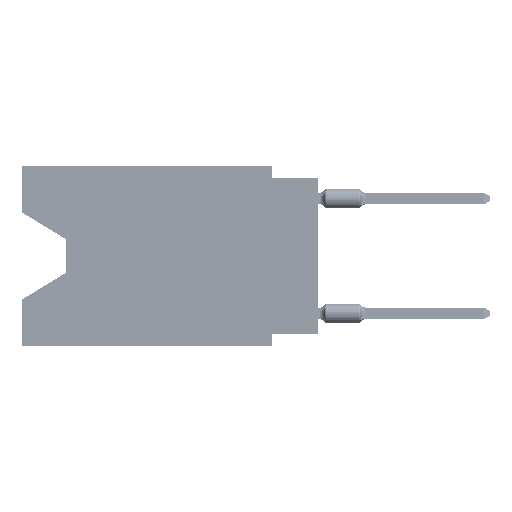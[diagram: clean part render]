
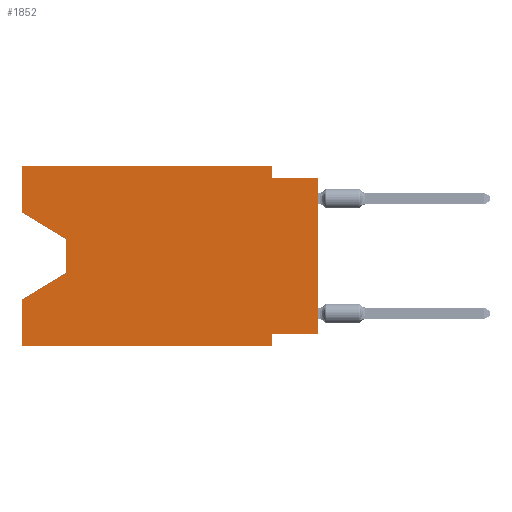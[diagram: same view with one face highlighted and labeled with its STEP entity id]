
A CAD part, left-side view. The second image highlights one B-rep face of the part: STEP entity #1852.
In plain terms, the highlighted planar face has unit normal (-1, 0, 0).
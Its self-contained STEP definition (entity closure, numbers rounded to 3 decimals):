
#822 = ORIENTED_EDGE ( 'NONE', *, *, #31095, .T. ) ;
#990 = CARTESIAN_POINT ( 'NONE',  ( 0., 16.383, 0. ) ) ;
#1060 = EDGE_CURVE ( 'NONE', #25016, #70449, #39018, .T. ) ;
#1229 = ORIENTED_EDGE ( 'NONE', *, *, #8433, .F. ) ;
#1852 = ADVANCED_FACE ( 'NONE', ( #47980 ), #70160, .F. ) ;
#2499 = ORIENTED_EDGE ( 'NONE', *, *, #43273, .F. ) ;
#2835 = EDGE_CURVE ( 'NONE', #46178, #70449, #46001, .T. ) ;
#5629 = ORIENTED_EDGE ( 'NONE', *, *, #1060, .F. ) ;
#6577 = DIRECTION ( 'NONE',  ( 0., -1., 0. ) ) ;
#7073 = EDGE_CURVE ( 'NONE', #48018, #15986, #58501, .T. ) ;
#8433 = EDGE_CURVE ( 'NONE', #41950, #25016, #15344, .T. ) ;
#8598 = VECTOR ( 'NONE', #38591, 1000. ) ;
#8704 = DIRECTION ( 'NONE',  ( 0., -1., 0. ) ) ;
#10518 = CARTESIAN_POINT ( 'NONE',  ( 0., 16.383, 0. ) ) ;
#12335 = VERTEX_POINT ( 'NONE', #43692 ) ;
#13188 = CARTESIAN_POINT ( 'NONE',  ( 0., 16.383, -2.546 ) ) ;
#13971 = ORIENTED_EDGE ( 'NONE', *, *, #64908, .F. ) ;
#14072 = CARTESIAN_POINT ( 'NONE',  ( 0., 2.54, -9.906 ) ) ;
#14372 = VERTEX_POINT ( 'NONE', #65568 ) ;
#14625 = DIRECTION ( 'NONE',  ( 0., 1., 0. ) ) ;
#14948 = CARTESIAN_POINT ( 'NONE',  ( 0., 13.97, -4.013 ) ) ;
#15196 = CARTESIAN_POINT ( 'NONE',  ( 0., 0., -9.271 ) ) ;
#15344 = LINE ( 'NONE', #53143, #36620 ) ;
#15986 = VERTEX_POINT ( 'NONE', #57147 ) ;
#16194 = ORIENTED_EDGE ( 'NONE', *, *, #7073, .F. ) ;
#17144 = ORIENTED_EDGE ( 'NONE', *, *, #54822, .T. ) ;
#17382 = DIRECTION ( 'NONE',  ( 0., 0., 1. ) ) ;
#17681 = DIRECTION ( 'NONE',  ( 0., 0., 1. ) ) ;
#18963 = VECTOR ( 'NONE', #17681, 1000. ) ;
#19224 = VECTOR ( 'NONE', #69356, 1000. ) ;
#20285 = VECTOR ( 'NONE', #48889, 1000. ) ;
#21452 = EDGE_CURVE ( 'NONE', #12335, #45288, #43662, .T. ) ;
#22569 = CARTESIAN_POINT ( 'NONE',  ( 0., 16.383, 0. ) ) ;
#22991 = CARTESIAN_POINT ( 'NONE',  ( 0., 2.54, 0. ) ) ;
#25016 = VERTEX_POINT ( 'NONE', #71754 ) ;
#25036 = VECTOR ( 'NONE', #8704, 1000. ) ;
#26215 = LINE ( 'NONE', #14948, #28585 ) ;
#27399 = ORIENTED_EDGE ( 'NONE', *, *, #30727, .T. ) ;
#28585 = VECTOR ( 'NONE', #48374, 1000. ) ;
#28944 = CARTESIAN_POINT ( 'NONE',  ( 0., 16.383, -9.906 ) ) ;
#29575 = CARTESIAN_POINT ( 'NONE',  ( 0., 2.54, -9.906 ) ) ;
#29761 = LINE ( 'NONE', #31193, #19224 ) ;
#30727 = EDGE_CURVE ( 'NONE', #41950, #15986, #54342, .T. ) ;
#31095 = EDGE_CURVE ( 'NONE', #48826, #69451, #36443, .T. ) ;
#31193 = CARTESIAN_POINT ( 'NONE',  ( 0., 13.97, -5.893 ) ) ;
#31634 = DIRECTION ( 'NONE',  ( 0., 0., -1. ) ) ;
#32834 = EDGE_CURVE ( 'NONE', #69451, #38051, #26215, .T. ) ;
#36196 = EDGE_LOOP ( 'NONE', ( #822, #46375, #17144, #2499, #64024, #5629, #1229, #27399, #16194, #13971, #56363, #38652 ) ) ;
#36443 = LINE ( 'NONE', #58630, #63208 ) ;
#36620 = VECTOR ( 'NONE', #14625, 1000. ) ;
#38051 = VERTEX_POINT ( 'NONE', #55431 ) ;
#38591 = DIRECTION ( 'NONE',  ( 0., 0., -1. ) ) ;
#38652 = ORIENTED_EDGE ( 'NONE', *, *, #53587, .F. ) ;
#39018 = LINE ( 'NONE', #29575, #42906 ) ;
#39137 = LINE ( 'NONE', #990, #18963 ) ;
#41950 = VERTEX_POINT ( 'NONE', #15196 ) ;
#42129 = CARTESIAN_POINT ( 'NONE',  ( 0., 0., -0.635 ) ) ;
#42344 = CARTESIAN_POINT ( 'NONE',  ( 0., 0., 0. ) ) ;
#42519 = CARTESIAN_POINT ( 'NONE',  ( 0., 16.383, 0. ) ) ;
#42906 = VECTOR ( 'NONE', #44831, 1000. ) ;
#43273 = EDGE_CURVE ( 'NONE', #46178, #14372, #39137, .T. ) ;
#43662 = LINE ( 'NONE', #22569, #67123 ) ;
#43692 = CARTESIAN_POINT ( 'NONE',  ( 0., 16.383, 0. ) ) ;
#43700 = LINE ( 'NONE', #60435, #8598 ) ;
#44639 = LINE ( 'NONE', #10518, #59856 ) ;
#44831 = DIRECTION ( 'NONE',  ( 0., 0., -1. ) ) ;
#45288 = VERTEX_POINT ( 'NONE', #22991 ) ;
#46001 = LINE ( 'NONE', #28944, #59492 ) ;
#46178 = VERTEX_POINT ( 'NONE', #57545 ) ;
#46375 = ORIENTED_EDGE ( 'NONE', *, *, #32834, .T. ) ;
#47980 = FACE_OUTER_BOUND ( 'NONE', #36196, .T. ) ;
#48018 = VERTEX_POINT ( 'NONE', #49649 ) ;
#48374 = DIRECTION ( 'NONE',  ( 0., 0., -1. ) ) ;
#48826 = VERTEX_POINT ( 'NONE', #13188 ) ;
#48889 = DIRECTION ( 'NONE',  ( 0., 0., 1. ) ) ;
#49649 = CARTESIAN_POINT ( 'NONE',  ( 0., 2.54, -0.635 ) ) ;
#53143 = CARTESIAN_POINT ( 'NONE',  ( 0., 0., -9.271 ) ) ;
#53587 = EDGE_CURVE ( 'NONE', #48826, #12335, #44639, .T. ) ;
#54342 = LINE ( 'NONE', #42344, #20285 ) ;
#54822 = EDGE_CURVE ( 'NONE', #38051, #14372, #29761, .T. ) ;
#55431 = CARTESIAN_POINT ( 'NONE',  ( 0., 13.97, -5.893 ) ) ;
#55803 = CARTESIAN_POINT ( 'NONE',  ( 0., 13.97, -4.013 ) ) ;
#56363 = ORIENTED_EDGE ( 'NONE', *, *, #21452, .F. ) ;
#57147 = CARTESIAN_POINT ( 'NONE',  ( 0., 0., -0.635 ) ) ;
#57545 = CARTESIAN_POINT ( 'NONE',  ( 0., 16.383, -9.906 ) ) ;
#58501 = LINE ( 'NONE', #42129, #25036 ) ;
#58630 = CARTESIAN_POINT ( 'NONE',  ( 0., 16.383, -2.546 ) ) ;
#59260 = DIRECTION ( 'NONE',  ( 1., 0., 0. ) ) ;
#59492 = VECTOR ( 'NONE', #68183, 1000. ) ;
#59856 = VECTOR ( 'NONE', #17382, 1000. ) ;
#60435 = CARTESIAN_POINT ( 'NONE',  ( 0., 2.54, 0. ) ) ;
#63208 = VECTOR ( 'NONE', #64813, 1000. ) ;
#64024 = ORIENTED_EDGE ( 'NONE', *, *, #2835, .T. ) ;
#64813 = DIRECTION ( 'NONE',  ( 0., -0.855, -0.519 ) ) ;
#64908 = EDGE_CURVE ( 'NONE', #45288, #48018, #43700, .T. ) ;
#65568 = CARTESIAN_POINT ( 'NONE',  ( 0., 16.383, -7.36 ) ) ;
#67123 = VECTOR ( 'NONE', #6577, 1000. ) ;
#68183 = DIRECTION ( 'NONE',  ( 0., -1., 0. ) ) ;
#69356 = DIRECTION ( 'NONE',  ( 0., 0.855, -0.519 ) ) ;
#69451 = VERTEX_POINT ( 'NONE', #55803 ) ;
#70160 = PLANE ( 'NONE',  #71016 ) ;
#70449 = VERTEX_POINT ( 'NONE', #14072 ) ;
#71016 = AXIS2_PLACEMENT_3D ( 'NONE', #42519, #59260, #31634 ) ;
#71754 = CARTESIAN_POINT ( 'NONE',  ( 0., 2.54, -9.271 ) ) ;
